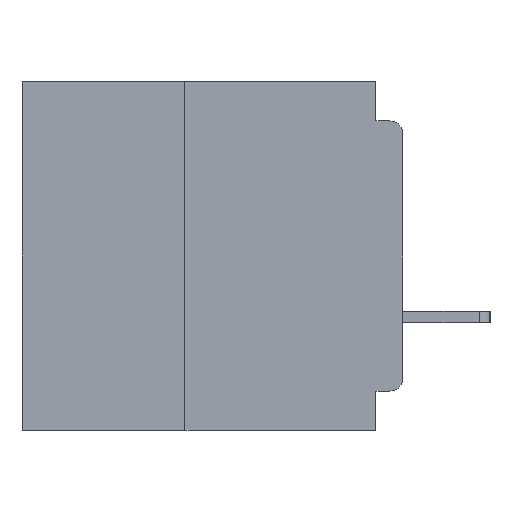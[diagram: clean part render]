
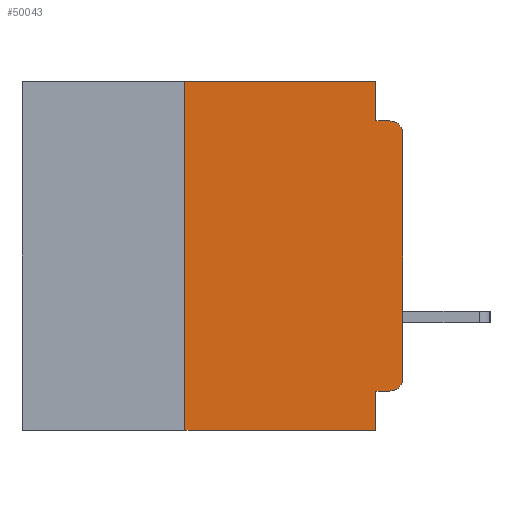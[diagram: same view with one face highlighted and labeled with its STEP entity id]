
A CAD part, left-side view. The second image highlights one B-rep face of the part: STEP entity #50043.
In plain terms, the highlighted planar face has unit normal (-1, 0, 0).
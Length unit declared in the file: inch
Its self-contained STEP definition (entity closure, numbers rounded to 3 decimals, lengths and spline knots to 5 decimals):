
#718 = VECTOR ( 'NONE', #12730, 39.37008 ) ;
#720 = ORIENTED_EDGE ( 'NONE', *, *, #33453, .F. ) ;
#4135 = DIRECTION ( 'NONE',  ( 0., 1., 0. ) ) ;
#4336 = VECTOR ( 'NONE', #51235, 39.37008 ) ;
#4872 = CARTESIAN_POINT ( 'NONE',  ( 0., 0., -0.34 ) ) ;
#5498 = DIRECTION ( 'NONE',  ( -1., 0., 0. ) ) ;
#5631 = VECTOR ( 'NONE', #28768, 39.37008 ) ;
#7322 = EDGE_CURVE ( 'NONE', #48328, #40646, #28278, .T. ) ;
#7465 = ORIENTED_EDGE ( 'NONE', *, *, #7322, .T. ) ;
#8143 = AXIS2_PLACEMENT_3D ( 'NONE', #33295, #5498, #37956 ) ;
#8442 = EDGE_CURVE ( 'NONE', #11070, #47882, #21585, .T. ) ;
#8938 = ORIENTED_EDGE ( 'NONE', *, *, #51642, .T. ) ;
#8965 = LINE ( 'NONE', #49756, #56783 ) ;
#9259 = ORIENTED_EDGE ( 'NONE', *, *, #8442, .F. ) ;
#11070 = VERTEX_POINT ( 'NONE', #43849 ) ;
#11403 = VECTOR ( 'NONE', #59640, 39.37008 ) ;
#11708 = VERTEX_POINT ( 'NONE', #20796 ) ;
#11751 = CIRCLE ( 'NONE', #31911, 0.015 ) ;
#12587 = DIRECTION ( 'NONE',  ( 0., 0., -1. ) ) ;
#12730 = DIRECTION ( 'NONE',  ( 0., 0., 1. ) ) ;
#12964 = DIRECTION ( 'NONE',  ( -1., 0., 0. ) ) ;
#14089 = CARTESIAN_POINT ( 'NONE',  ( 0., 0.437, -0.4 ) ) ;
#15158 = PLANE ( 'NONE',  #37701 ) ;
#16598 = CARTESIAN_POINT ( 'NONE',  ( 0., 0.031, -0.4 ) ) ;
#17219 = CIRCLE ( 'NONE', #8143, 0.015 ) ;
#19825 = DIRECTION ( 'NONE',  ( 1., 0., 0. ) ) ;
#20048 = DIRECTION ( 'NONE',  ( 0., 0., 1. ) ) ;
#20210 = EDGE_LOOP ( 'NONE', ( #7465, #8938, #720, #49955, #33189, #9259, #53023, #57912, #32169, #51258 ) ) ;
#20796 = CARTESIAN_POINT ( 'NONE',  ( 0., 0.015, -0.355 ) ) ;
#20834 = LINE ( 'NONE', #24095, #5631 ) ;
#21585 = LINE ( 'NONE', #52538, #44882 ) ;
#24095 = CARTESIAN_POINT ( 'NONE',  ( 0., 0.437, 0. ) ) ;
#26274 = VERTEX_POINT ( 'NONE', #40718 ) ;
#26445 = EDGE_CURVE ( 'NONE', #11070, #43361, #55118, .T. ) ;
#28278 = LINE ( 'NONE', #45232, #718 ) ;
#28426 = VERTEX_POINT ( 'NONE', #59987 ) ;
#28550 = EDGE_CURVE ( 'NONE', #11708, #48328, #17219, .T. ) ;
#28768 = DIRECTION ( 'NONE',  ( 0., -1., 0. ) ) ;
#29364 = FACE_OUTER_BOUND ( 'NONE', #20210, .T. ) ;
#29838 = VECTOR ( 'NONE', #4135, 39.37008 ) ;
#31911 = AXIS2_PLACEMENT_3D ( 'NONE', #40798, #12964, #45478 ) ;
#31938 = CARTESIAN_POINT ( 'NONE',  ( 0., 0., -0.355 ) ) ;
#32169 = ORIENTED_EDGE ( 'NONE', *, *, #36551, .F. ) ;
#33189 = ORIENTED_EDGE ( 'NONE', *, *, #44937, .F. ) ;
#33295 = CARTESIAN_POINT ( 'NONE',  ( 0., 0.015, -0.34 ) ) ;
#33453 = EDGE_CURVE ( 'NONE', #55807, #26274, #36095, .T. ) ;
#36095 = LINE ( 'NONE', #55011, #11403 ) ;
#36551 = EDGE_CURVE ( 'NONE', #11708, #28426, #54515, .T. ) ;
#36555 = CARTESIAN_POINT ( 'NONE',  ( 0., 0., -0.06 ) ) ;
#36968 = LINE ( 'NONE', #16598, #57229 ) ;
#37077 = EDGE_CURVE ( 'NONE', #57616, #55807, #8965, .T. ) ;
#37701 = AXIS2_PLACEMENT_3D ( 'NONE', #43022, #19825, #52301 ) ;
#37956 = DIRECTION ( 'NONE',  ( 0., 0., -1. ) ) ;
#40646 = VERTEX_POINT ( 'NONE', #36555 ) ;
#40718 = CARTESIAN_POINT ( 'NONE',  ( 0., 0.015, -0.045 ) ) ;
#40798 = CARTESIAN_POINT ( 'NONE',  ( 0., 0.015, -0.06 ) ) ;
#43022 = CARTESIAN_POINT ( 'NONE',  ( 0., 0.437, 0. ) ) ;
#43291 = CARTESIAN_POINT ( 'NONE',  ( 0., 0.25, 0. ) ) ;
#43361 = VERTEX_POINT ( 'NONE', #54830 ) ;
#43849 = CARTESIAN_POINT ( 'NONE',  ( 0., 0.25, -0.4 ) ) ;
#44882 = VECTOR ( 'NONE', #20048, 39.37008 ) ;
#44937 = EDGE_CURVE ( 'NONE', #47882, #57616, #20834, .T. ) ;
#45232 = CARTESIAN_POINT ( 'NONE',  ( 0., 0., 0. ) ) ;
#45478 = DIRECTION ( 'NONE',  ( 0., 0., -1. ) ) ;
#47882 = VERTEX_POINT ( 'NONE', #43291 ) ;
#48328 = VERTEX_POINT ( 'NONE', #4872 ) ;
#49756 = CARTESIAN_POINT ( 'NONE',  ( 0., 0.031, 0. ) ) ;
#49955 = ORIENTED_EDGE ( 'NONE', *, *, #37077, .F. ) ;
#50043 = ADVANCED_FACE ( 'NONE', ( #29364 ), #15158, .F. ) ;
#50678 = CARTESIAN_POINT ( 'NONE',  ( 0., 0.031, 0. ) ) ;
#51078 = CARTESIAN_POINT ( 'NONE',  ( 0., 0.031, -0.045 ) ) ;
#51235 = DIRECTION ( 'NONE',  ( 0., -1., 0. ) ) ;
#51258 = ORIENTED_EDGE ( 'NONE', *, *, #28550, .T. ) ;
#51642 = EDGE_CURVE ( 'NONE', #40646, #26274, #11751, .T. ) ;
#52301 = DIRECTION ( 'NONE',  ( 0., 0., -1. ) ) ;
#52538 = CARTESIAN_POINT ( 'NONE',  ( 0., 0.25, -0.4 ) ) ;
#53023 = ORIENTED_EDGE ( 'NONE', *, *, #26445, .T. ) ;
#53717 = DIRECTION ( 'NONE',  ( 0., 0., -1. ) ) ;
#53772 = EDGE_CURVE ( 'NONE', #28426, #43361, #36968, .T. ) ;
#54515 = LINE ( 'NONE', #31938, #29838 ) ;
#54830 = CARTESIAN_POINT ( 'NONE',  ( 0., 0.031, -0.4 ) ) ;
#55011 = CARTESIAN_POINT ( 'NONE',  ( 0., 0., -0.045 ) ) ;
#55118 = LINE ( 'NONE', #14089, #4336 ) ;
#55807 = VERTEX_POINT ( 'NONE', #51078 ) ;
#56783 = VECTOR ( 'NONE', #12587, 39.37008 ) ;
#57229 = VECTOR ( 'NONE', #53717, 39.37008 ) ;
#57616 = VERTEX_POINT ( 'NONE', #50678 ) ;
#57912 = ORIENTED_EDGE ( 'NONE', *, *, #53772, .F. ) ;
#59640 = DIRECTION ( 'NONE',  ( 0., -1., 0. ) ) ;
#59987 = CARTESIAN_POINT ( 'NONE',  ( 0., 0.031, -0.355 ) ) ;
